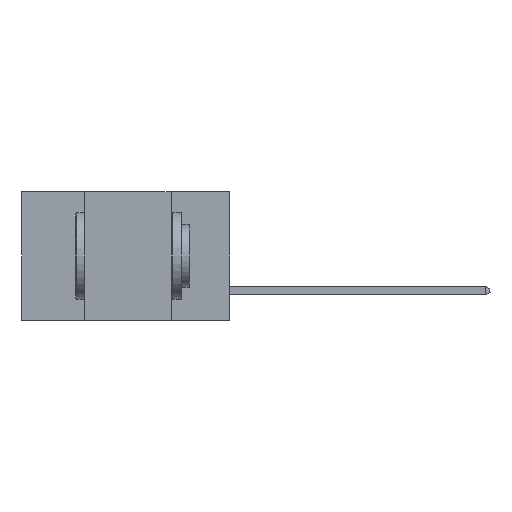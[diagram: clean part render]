
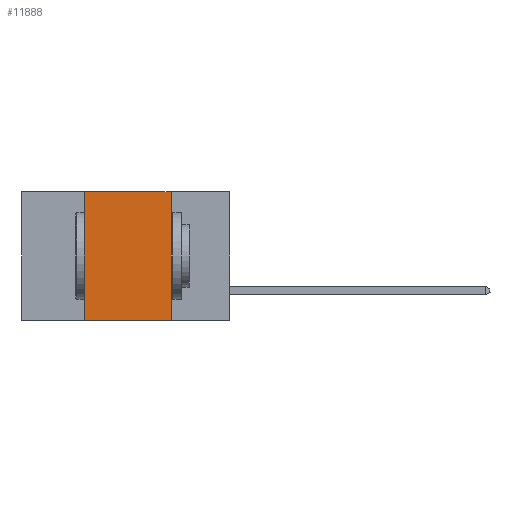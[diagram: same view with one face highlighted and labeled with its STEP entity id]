
A CAD part, left-side view. The second image highlights one B-rep face of the part: STEP entity #11888.
In plain terms, the highlighted planar face has unit normal (-1, 0, 0).
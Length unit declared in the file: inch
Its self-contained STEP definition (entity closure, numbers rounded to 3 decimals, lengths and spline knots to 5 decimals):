
#823 = CARTESIAN_POINT ( 'NONE',  ( 0., 0.17, 0. ) ) ;
#835 = CARTESIAN_POINT ( 'NONE',  ( 0., 0.42, -0.37 ) ) ;
#1468 = DIRECTION ( 'NONE',  ( 0., -1., 0. ) ) ;
#2444 = DIRECTION ( 'NONE',  ( 0., -1., 0. ) ) ;
#2453 = FACE_OUTER_BOUND ( 'NONE', #12339, .T. ) ;
#2592 = VERTEX_POINT ( 'NONE', #835 ) ;
#3886 = CARTESIAN_POINT ( 'NONE',  ( 0., 0.42, 0. ) ) ;
#4080 = CARTESIAN_POINT ( 'NONE',  ( 0., 0.6, 0. ) ) ;
#4165 = CARTESIAN_POINT ( 'NONE',  ( 0., 0.17, 0. ) ) ;
#5710 = VECTOR ( 'NONE', #2444, 39.37008 ) ;
#5751 = CARTESIAN_POINT ( 'NONE',  ( 0., 0.17, -0.37 ) ) ;
#6203 = EDGE_CURVE ( 'NONE', #2592, #12103, #6835, .T. ) ;
#6760 = DIRECTION ( 'NONE',  ( 0., 0., -1. ) ) ;
#6835 = LINE ( 'NONE', #12546, #5710 ) ;
#7320 = DIRECTION ( 'NONE',  ( 0., 0., -1. ) ) ;
#7433 = ORIENTED_EDGE ( 'NONE', *, *, #6203, .T. ) ;
#7682 = VECTOR ( 'NONE', #8225, 39.37008 ) ;
#7830 = PLANE ( 'NONE',  #7912 ) ;
#7912 = AXIS2_PLACEMENT_3D ( 'NONE', #13651, #9634, #6760 ) ;
#7926 = VERTEX_POINT ( 'NONE', #14796 ) ;
#8225 = DIRECTION ( 'NONE',  ( 0., 0., 1. ) ) ;
#8241 = ORIENTED_EDGE ( 'NONE', *, *, #18142, .F. ) ;
#9634 = DIRECTION ( 'NONE',  ( 1., 0., 0. ) ) ;
#11370 = EDGE_CURVE ( 'NONE', #17363, #12103, #11637, .T. ) ;
#11637 = LINE ( 'NONE', #4165, #16993 ) ;
#11888 = ADVANCED_FACE ( 'NONE', ( #2453 ), #7830, .F. ) ;
#12103 = VERTEX_POINT ( 'NONE', #5751 ) ;
#12326 = ORIENTED_EDGE ( 'NONE', *, *, #11370, .F. ) ;
#12339 = EDGE_LOOP ( 'NONE', ( #12326, #15262, #8241, #7433 ) ) ;
#12433 = EDGE_CURVE ( 'NONE', #7926, #17363, #15587, .T. ) ;
#12546 = CARTESIAN_POINT ( 'NONE',  ( 0., 0.6, -0.37 ) ) ;
#12920 = VECTOR ( 'NONE', #1468, 39.37008 ) ;
#13651 = CARTESIAN_POINT ( 'NONE',  ( 0., 0.6, 0. ) ) ;
#14796 = CARTESIAN_POINT ( 'NONE',  ( 0., 0.42, 0. ) ) ;
#15262 = ORIENTED_EDGE ( 'NONE', *, *, #12433, .F. ) ;
#15587 = LINE ( 'NONE', #4080, #12920 ) ;
#16518 = LINE ( 'NONE', #3886, #7682 ) ;
#16993 = VECTOR ( 'NONE', #7320, 39.37008 ) ;
#17363 = VERTEX_POINT ( 'NONE', #823 ) ;
#18142 = EDGE_CURVE ( 'NONE', #2592, #7926, #16518, .T. ) ;
